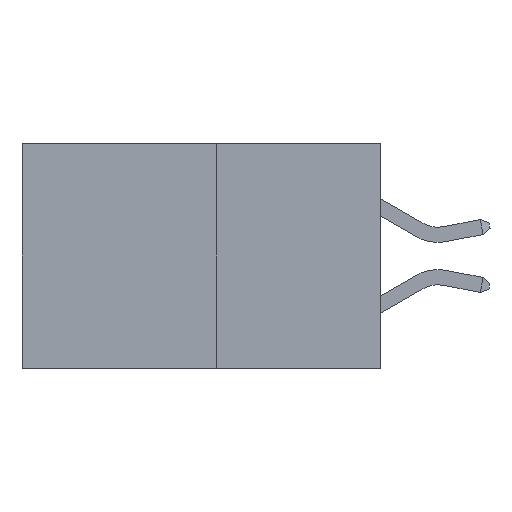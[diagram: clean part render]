
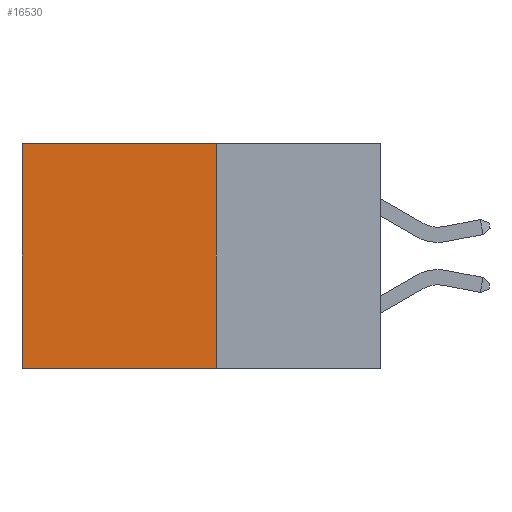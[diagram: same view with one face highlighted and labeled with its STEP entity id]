
A CAD part, left-side view. The second image highlights one B-rep face of the part: STEP entity #16530.
In plain terms, the highlighted planar face has unit normal (-1, 0, 0).
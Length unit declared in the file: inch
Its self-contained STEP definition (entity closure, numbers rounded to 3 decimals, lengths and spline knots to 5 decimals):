
#910 = EDGE_CURVE ( 'NONE', #9333, #12254, #17868, .T. ) ;
#2712 = ORIENTED_EDGE ( 'NONE', *, *, #13048, .F. ) ;
#3007 = CARTESIAN_POINT ( 'NONE',  ( 0.277, 0.27, 0. ) ) ;
#3313 = LINE ( 'NONE', #10161, #13801 ) ;
#3421 = VECTOR ( 'NONE', #13959, 39.37008 ) ;
#3552 = EDGE_CURVE ( 'NONE', #4464, #16986, #5529, .T. ) ;
#3770 = DIRECTION ( 'NONE',  ( 0., 0., -1. ) ) ;
#4050 = ORIENTED_EDGE ( 'NONE', *, *, #15877, .T. ) ;
#4464 = VERTEX_POINT ( 'NONE', #4768 ) ;
#4768 = CARTESIAN_POINT ( 'NONE',  ( 0.277, 0.27, 0. ) ) ;
#5529 = LINE ( 'NONE', #6630, #15572 ) ;
#5697 = PLANE ( 'NONE',  #14670 ) ;
#5789 = CARTESIAN_POINT ( 'NONE',  ( 0.277, 0.59, -0.37 ) ) ;
#6630 = CARTESIAN_POINT ( 'NONE',  ( 0.277, 0.27, -0.37 ) ) ;
#7010 = DIRECTION ( 'NONE',  ( 0., 0., -1. ) ) ;
#8287 = CARTESIAN_POINT ( 'NONE',  ( 0.277, 0.27, -0.37 ) ) ;
#8430 = FACE_OUTER_BOUND ( 'NONE', #13911, .T. ) ;
#9333 = VERTEX_POINT ( 'NONE', #9796 ) ;
#9796 = CARTESIAN_POINT ( 'NONE',  ( 0.277, 0.59, 0. ) ) ;
#10161 = CARTESIAN_POINT ( 'NONE',  ( 0.277, 0.27, -0.37 ) ) ;
#10471 = CARTESIAN_POINT ( 'NONE',  ( 0.277, 0.27, -0.37 ) ) ;
#12254 = VERTEX_POINT ( 'NONE', #12935 ) ;
#12935 = CARTESIAN_POINT ( 'NONE',  ( 0.277, 0.59, -0.37 ) ) ;
#13048 = EDGE_CURVE ( 'NONE', #16986, #12254, #3313, .T. ) ;
#13801 = VECTOR ( 'NONE', #15715, 39.37008 ) ;
#13911 = EDGE_LOOP ( 'NONE', ( #15558, #2712, #14496, #4050 ) ) ;
#13959 = DIRECTION ( 'NONE',  ( 0., 1., 0. ) ) ;
#14496 = ORIENTED_EDGE ( 'NONE', *, *, #3552, .F. ) ;
#14670 = AXIS2_PLACEMENT_3D ( 'NONE', #8287, #15251, #7010 ) ;
#15251 = DIRECTION ( 'NONE',  ( 1., 0., 0. ) ) ;
#15558 = ORIENTED_EDGE ( 'NONE', *, *, #910, .T. ) ;
#15572 = VECTOR ( 'NONE', #16078, 39.37008 ) ;
#15715 = DIRECTION ( 'NONE',  ( 0., 1., 0. ) ) ;
#15877 = EDGE_CURVE ( 'NONE', #4464, #9333, #17780, .T. ) ;
#16078 = DIRECTION ( 'NONE',  ( 0., 0., -1. ) ) ;
#16530 = ADVANCED_FACE ( 'NONE', ( #8430 ), #5697, .F. ) ;
#16986 = VERTEX_POINT ( 'NONE', #10471 ) ;
#17475 = VECTOR ( 'NONE', #3770, 39.37008 ) ;
#17780 = LINE ( 'NONE', #3007, #3421 ) ;
#17868 = LINE ( 'NONE', #5789, #17475 ) ;
